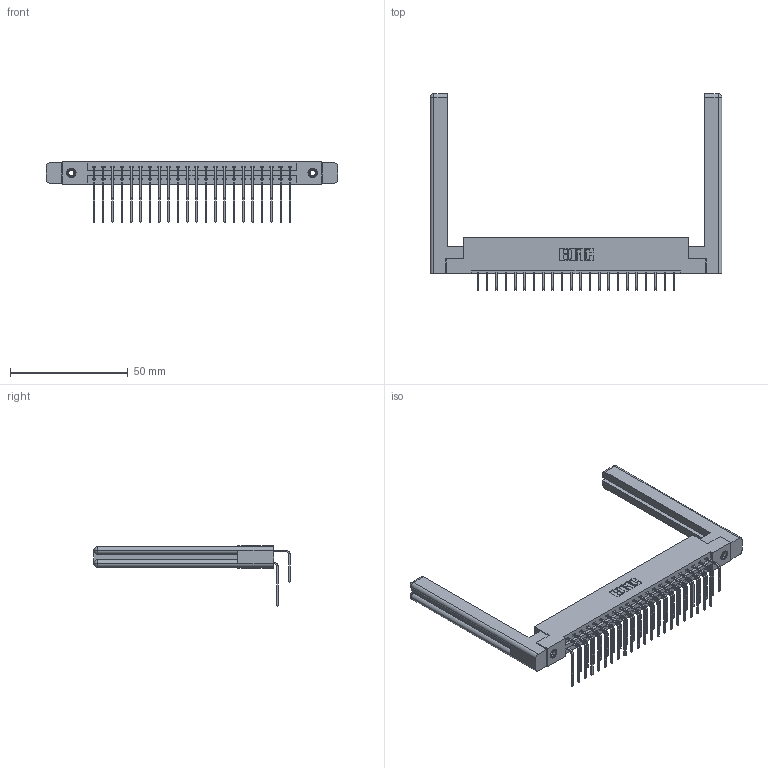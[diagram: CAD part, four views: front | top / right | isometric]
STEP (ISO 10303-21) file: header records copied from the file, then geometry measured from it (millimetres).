
FILE_DESCRIPTION (( 'STEP AP203' ), '1' );
FILE_NAME ('337-044-558-258.STEP', '2019-10-09T13:24:20', ( '' ), ( '' ), 'SwSTEP 2.0', 'SolidWorks 2016', '' );
FILE_SCHEMA (( 'CONFIG_CONTROL_DESIGN' ));
Length unit declared in the file: inch
Products named in the file (6): 337 Part_Flush Mounting Lugs - 0.156 Dia-TI; 337-044-558-258; 307-220-058; 345-292-001_558 Tail - 2; 345-292-001_558 559 Tail - 1; 345-250-001_345-250-001-102
Assembly tree (49 placements, depth 2):
  337-044-558-258
    337 Part_Flush Mounting Lugs - 0.156 Dia-TI
    345-292-001_558 559 Tail - 1  x22
    345-292-001_558 Tail - 2  x22
    345-250-001_345-250-001-102  x2
    307-220-058  x2
Bounding box: 123.8 x 83.25 x 25.53 mm (x, y, z)
Volume: 20176.9 mm3; surface area: 20862.6 mm2
Topology: 49 solids, 49 shells, 2720 faces, 8013 edges, 5270 vertices
Faces by surface type: plane 1914, cylinder 782, cone 12, torus 12
Entity records: 24062 total; most frequent: CARTESIAN_POINT 4124, ORIENTED_EDGE 3948, DIRECTION 3542, EDGE_CURVE 1974, LINE 1758, VECTOR 1758, VERTEX_POINT 1306, AXIS2_PLACEMENT_3D 892
